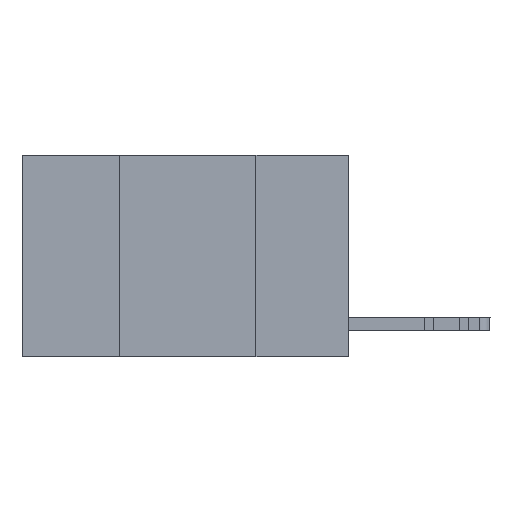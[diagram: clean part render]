
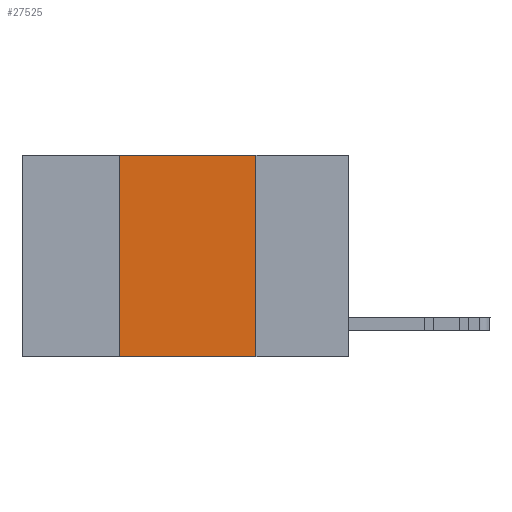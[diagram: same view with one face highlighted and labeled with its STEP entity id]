
A CAD part, left-side view. The second image highlights one B-rep face of the part: STEP entity #27525.
In plain terms, the highlighted planar face has unit normal (-1, 0, 0).
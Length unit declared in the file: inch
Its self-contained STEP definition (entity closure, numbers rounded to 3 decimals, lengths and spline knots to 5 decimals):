
#314 = VECTOR ( 'NONE', #19224, 39.37008 ) ;
#1046 = LINE ( 'NONE', #17001, #314 ) ;
#1484 = CARTESIAN_POINT ( 'NONE',  ( 0., 0.6, -0.37 ) ) ;
#1832 = DIRECTION ( 'NONE',  ( 1., 0., 0. ) ) ;
#3185 = EDGE_CURVE ( 'NONE', #21128, #23674, #1046, .T. ) ;
#5116 = LINE ( 'NONE', #18134, #10447 ) ;
#6487 = CARTESIAN_POINT ( 'NONE',  ( 0., 0.6, 0. ) ) ;
#8037 = VECTOR ( 'NONE', #24032, 39.37008 ) ;
#8776 = PLANE ( 'NONE',  #29061 ) ;
#9314 = EDGE_CURVE ( 'NONE', #21128, #13165, #16860, .T. ) ;
#10447 = VECTOR ( 'NONE', #28455, 39.37008 ) ;
#10957 = CARTESIAN_POINT ( 'NONE',  ( 0., 0.17, -0.37 ) ) ;
#11028 = DIRECTION ( 'NONE',  ( 0., 0., -1. ) ) ;
#11125 = ORIENTED_EDGE ( 'NONE', *, *, #9314, .T. ) ;
#11855 = CARTESIAN_POINT ( 'NONE',  ( 0., 0.17, 0. ) ) ;
#12862 = DIRECTION ( 'NONE',  ( 0., -1., 0. ) ) ;
#12897 = CARTESIAN_POINT ( 'NONE',  ( 0., 0.17, 0. ) ) ;
#12905 = VERTEX_POINT ( 'NONE', #11855 ) ;
#13165 = VERTEX_POINT ( 'NONE', #10957 ) ;
#13577 = ORIENTED_EDGE ( 'NONE', *, *, #3185, .F. ) ;
#15208 = CARTESIAN_POINT ( 'NONE',  ( 0., 0.42, -0.37 ) ) ;
#16860 = LINE ( 'NONE', #1484, #22070 ) ;
#17001 = CARTESIAN_POINT ( 'NONE',  ( 0., 0.42, 0. ) ) ;
#18134 = CARTESIAN_POINT ( 'NONE',  ( 0., 0.6, 0. ) ) ;
#19224 = DIRECTION ( 'NONE',  ( 0., 0., 1. ) ) ;
#19928 = LINE ( 'NONE', #12897, #8037 ) ;
#20836 = CARTESIAN_POINT ( 'NONE',  ( 0., 0.42, 0. ) ) ;
#21128 = VERTEX_POINT ( 'NONE', #15208 ) ;
#22070 = VECTOR ( 'NONE', #12862, 39.37008 ) ;
#22251 = EDGE_CURVE ( 'NONE', #12905, #13165, #19928, .T. ) ;
#22636 = ORIENTED_EDGE ( 'NONE', *, *, #22251, .F. ) ;
#23506 = EDGE_CURVE ( 'NONE', #23674, #12905, #5116, .T. ) ;
#23674 = VERTEX_POINT ( 'NONE', #20836 ) ;
#24032 = DIRECTION ( 'NONE',  ( 0., 0., -1. ) ) ;
#24064 = ORIENTED_EDGE ( 'NONE', *, *, #23506, .F. ) ;
#26565 = EDGE_LOOP ( 'NONE', ( #22636, #24064, #13577, #11125 ) ) ;
#27525 = ADVANCED_FACE ( 'NONE', ( #28188 ), #8776, .F. ) ;
#28188 = FACE_OUTER_BOUND ( 'NONE', #26565, .T. ) ;
#28455 = DIRECTION ( 'NONE',  ( 0., -1., 0. ) ) ;
#29061 = AXIS2_PLACEMENT_3D ( 'NONE', #6487, #1832, #11028 ) ;
